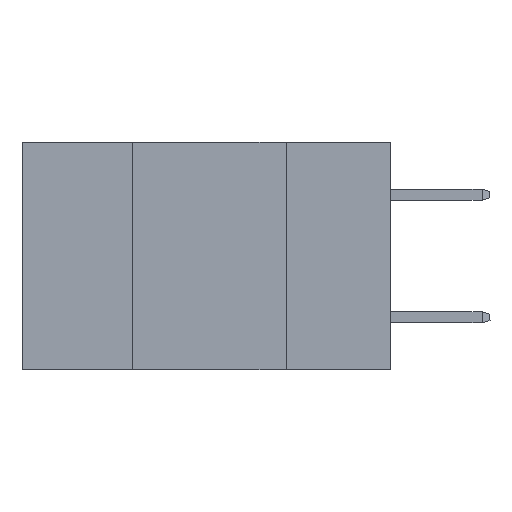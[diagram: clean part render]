
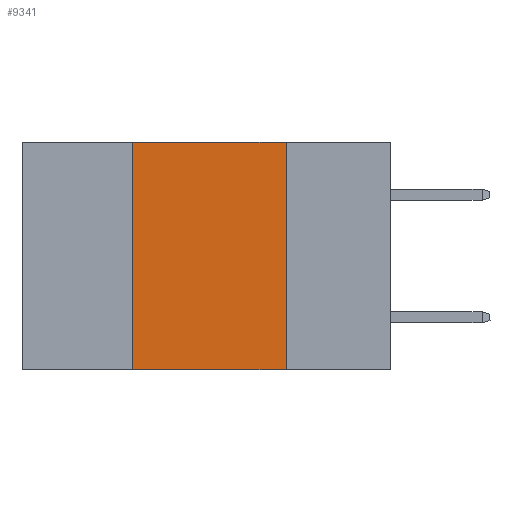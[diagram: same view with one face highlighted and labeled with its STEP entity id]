
A CAD part, left-side view. The second image highlights one B-rep face of the part: STEP entity #9341.
In plain terms, the highlighted planar face has unit normal (-1, 0, 0).
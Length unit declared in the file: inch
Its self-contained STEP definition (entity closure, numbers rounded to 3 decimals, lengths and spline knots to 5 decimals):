
#262 = CARTESIAN_POINT ( 'NONE',  ( 0., 0.42, 0. ) ) ;
#585 = CARTESIAN_POINT ( 'NONE',  ( 0., 0.6, 0. ) ) ;
#1037 = LINE ( 'NONE', #16911, #15771 ) ;
#1136 = CARTESIAN_POINT ( 'NONE',  ( 0., 0.42, -0.37 ) ) ;
#1163 = CARTESIAN_POINT ( 'NONE',  ( 0., 0.17, 0. ) ) ;
#1416 = ORIENTED_EDGE ( 'NONE', *, *, #14320, .F. ) ;
#1848 = VERTEX_POINT ( 'NONE', #1136 ) ;
#2298 = VECTOR ( 'NONE', #13749, 39.37008 ) ;
#2426 = EDGE_CURVE ( 'NONE', #1848, #12439, #8304, .T. ) ;
#2962 = CARTESIAN_POINT ( 'NONE',  ( 0., 0.6, 0. ) ) ;
#3010 = DIRECTION ( 'NONE',  ( 0., -1., 0. ) ) ;
#4379 = DIRECTION ( 'NONE',  ( 0., -1., 0. ) ) ;
#4506 = VECTOR ( 'NONE', #3010, 39.37008 ) ;
#5010 = CARTESIAN_POINT ( 'NONE',  ( 0., 0.17, 0. ) ) ;
#6065 = LINE ( 'NONE', #5010, #2298 ) ;
#6348 = PLANE ( 'NONE',  #10737 ) ;
#7030 = VERTEX_POINT ( 'NONE', #1163 ) ;
#7270 = EDGE_CURVE ( 'NONE', #9580, #7030, #17901, .T. ) ;
#7573 = EDGE_CURVE ( 'NONE', #7030, #12439, #6065, .T. ) ;
#7761 = DIRECTION ( 'NONE',  ( 1., 0., 0. ) ) ;
#8099 = CARTESIAN_POINT ( 'NONE',  ( 0., 0.17, -0.37 ) ) ;
#8304 = LINE ( 'NONE', #12997, #4506 ) ;
#8518 = ORIENTED_EDGE ( 'NONE', *, *, #7573, .F. ) ;
#8655 = FACE_OUTER_BOUND ( 'NONE', #16343, .T. ) ;
#9341 = ADVANCED_FACE ( 'NONE', ( #8655 ), #6348, .F. ) ;
#9580 = VERTEX_POINT ( 'NONE', #262 ) ;
#9944 = DIRECTION ( 'NONE',  ( 0., 0., 1. ) ) ;
#10737 = AXIS2_PLACEMENT_3D ( 'NONE', #585, #7761, #17563 ) ;
#12422 = ORIENTED_EDGE ( 'NONE', *, *, #7270, .F. ) ;
#12439 = VERTEX_POINT ( 'NONE', #8099 ) ;
#12997 = CARTESIAN_POINT ( 'NONE',  ( 0., 0.6, -0.37 ) ) ;
#13749 = DIRECTION ( 'NONE',  ( 0., 0., -1. ) ) ;
#14320 = EDGE_CURVE ( 'NONE', #1848, #9580, #1037, .T. ) ;
#15771 = VECTOR ( 'NONE', #9944, 39.37008 ) ;
#16343 = EDGE_LOOP ( 'NONE', ( #8518, #12422, #1416, #16520 ) ) ;
#16520 = ORIENTED_EDGE ( 'NONE', *, *, #2426, .T. ) ;
#16911 = CARTESIAN_POINT ( 'NONE',  ( 0., 0.42, 0. ) ) ;
#17493 = VECTOR ( 'NONE', #4379, 39.37008 ) ;
#17563 = DIRECTION ( 'NONE',  ( 0., 0., -1. ) ) ;
#17901 = LINE ( 'NONE', #2962, #17493 ) ;
